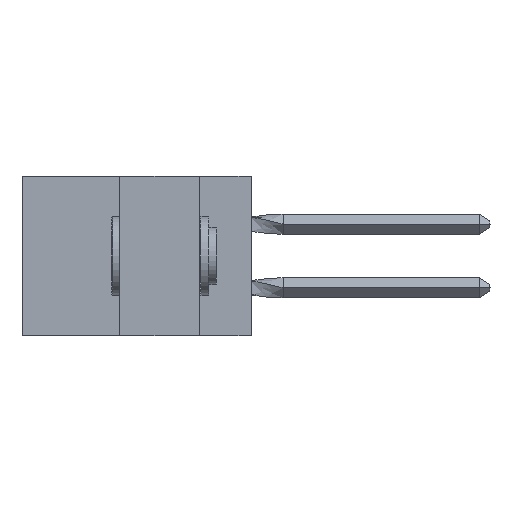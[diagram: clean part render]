
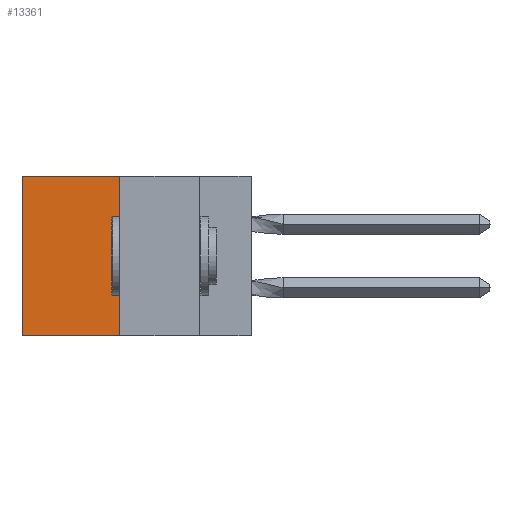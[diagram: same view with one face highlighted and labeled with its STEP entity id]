
A CAD part, left-side view. The second image highlights one B-rep face of the part: STEP entity #13361.
In plain terms, the highlighted planar face has unit normal (-1, 0, 0).
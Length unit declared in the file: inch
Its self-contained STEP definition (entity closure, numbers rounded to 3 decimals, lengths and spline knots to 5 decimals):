
#605 = CARTESIAN_POINT ( 'NONE',  ( 0.305, 0.413, -0.5 ) ) ;
#657 = DIRECTION ( 'NONE',  ( 0., 1., 0. ) ) ;
#728 = DIRECTION ( 'NONE',  ( 0., 1., 0. ) ) ;
#1772 = AXIS2_PLACEMENT_3D ( 'NONE', #605, #8182, #21813 ) ;
#1810 = VERTEX_POINT ( 'NONE', #21385 ) ;
#2477 = EDGE_CURVE ( 'NONE', #17487, #1810, #7560, .T. ) ;
#2821 = CARTESIAN_POINT ( 'NONE',  ( 0.305, 0.413, -0.5 ) ) ;
#4052 = FACE_OUTER_BOUND ( 'NONE', #12411, .T. ) ;
#4246 = PLANE ( 'NONE',  #1772 ) ;
#4348 = CARTESIAN_POINT ( 'NONE',  ( 0.305, 0.413, -0.5 ) ) ;
#7560 = LINE ( 'NONE', #2821, #18454 ) ;
#8115 = DIRECTION ( 'NONE',  ( 0., 0., -1. ) ) ;
#8182 = DIRECTION ( 'NONE',  ( 1., 0., 0. ) ) ;
#9088 = LINE ( 'NONE', #4348, #12400 ) ;
#9111 = ORIENTED_EDGE ( 'NONE', *, *, #16229, .T. ) ;
#10530 = CARTESIAN_POINT ( 'NONE',  ( 0.305, 0.72, -0.5 ) ) ;
#10602 = LINE ( 'NONE', #17962, #24838 ) ;
#11334 = ORIENTED_EDGE ( 'NONE', *, *, #2477, .F. ) ;
#11834 = VERTEX_POINT ( 'NONE', #12062 ) ;
#12062 = CARTESIAN_POINT ( 'NONE',  ( 0.305, 0.413, 0. ) ) ;
#12326 = VECTOR ( 'NONE', #12646, 39.37008 ) ;
#12400 = VECTOR ( 'NONE', #8115, 39.37008 ) ;
#12411 = EDGE_LOOP ( 'NONE', ( #9111, #11334, #14352, #20142 ) ) ;
#12646 = DIRECTION ( 'NONE',  ( 0., 0., -1. ) ) ;
#13361 = ADVANCED_FACE ( 'NONE', ( #4052 ), #4246, .F. ) ;
#14288 = CARTESIAN_POINT ( 'NONE',  ( 0.305, 0.72, 0. ) ) ;
#14352 = ORIENTED_EDGE ( 'NONE', *, *, #14907, .F. ) ;
#14715 = EDGE_CURVE ( 'NONE', #11834, #15851, #10602, .T. ) ;
#14907 = EDGE_CURVE ( 'NONE', #11834, #17487, #9088, .T. ) ;
#15190 = CARTESIAN_POINT ( 'NONE',  ( 0.305, 0.413, -0.5 ) ) ;
#15851 = VERTEX_POINT ( 'NONE', #14288 ) ;
#16229 = EDGE_CURVE ( 'NONE', #15851, #1810, #17496, .T. ) ;
#17487 = VERTEX_POINT ( 'NONE', #15190 ) ;
#17496 = LINE ( 'NONE', #10530, #12326 ) ;
#17962 = CARTESIAN_POINT ( 'NONE',  ( 0.305, 0.413, 0. ) ) ;
#18454 = VECTOR ( 'NONE', #657, 39.37008 ) ;
#20142 = ORIENTED_EDGE ( 'NONE', *, *, #14715, .T. ) ;
#21385 = CARTESIAN_POINT ( 'NONE',  ( 0.305, 0.72, -0.5 ) ) ;
#21813 = DIRECTION ( 'NONE',  ( 0., 0., -1. ) ) ;
#24838 = VECTOR ( 'NONE', #728, 39.37008 ) ;
